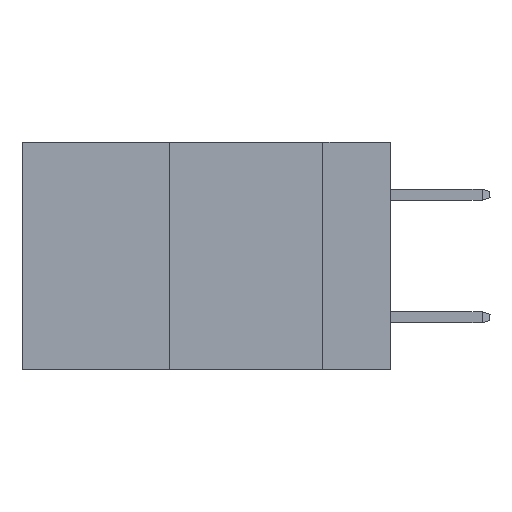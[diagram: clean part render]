
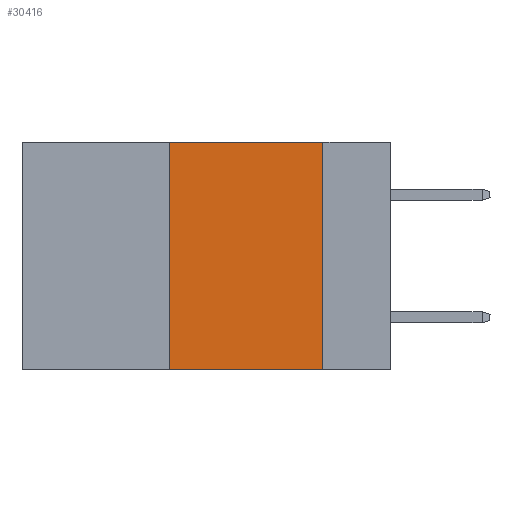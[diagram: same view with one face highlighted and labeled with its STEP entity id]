
A CAD part, left-side view. The second image highlights one B-rep face of the part: STEP entity #30416.
In plain terms, the highlighted planar face has unit normal (-1, 0, 0).
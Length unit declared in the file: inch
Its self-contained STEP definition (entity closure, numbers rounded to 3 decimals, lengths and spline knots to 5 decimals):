
#1868 = CARTESIAN_POINT ( 'NONE',  ( 0., 0.11, 0. ) ) ;
#5087 = DIRECTION ( 'NONE',  ( 1., 0., 0. ) ) ;
#5675 = CARTESIAN_POINT ( 'NONE',  ( 0., 0.6, 0. ) ) ;
#8680 = DIRECTION ( 'NONE',  ( 0., 0., -1. ) ) ;
#9244 = CARTESIAN_POINT ( 'NONE',  ( 0., 0.6, 0. ) ) ;
#10865 = DIRECTION ( 'NONE',  ( 0., -1., 0. ) ) ;
#11675 = ORIENTED_EDGE ( 'NONE', *, *, #19535, .T. ) ;
#11984 = DIRECTION ( 'NONE',  ( 0., 0., -1. ) ) ;
#12924 = ORIENTED_EDGE ( 'NONE', *, *, #38680, .F. ) ;
#15385 = VECTOR ( 'NONE', #33430, 39.37008 ) ;
#16258 = VERTEX_POINT ( 'NONE', #24837 ) ;
#16572 = EDGE_CURVE ( 'NONE', #40234, #34089, #17616, .T. ) ;
#17616 = LINE ( 'NONE', #18997, #23448 ) ;
#18564 = AXIS2_PLACEMENT_3D ( 'NONE', #5675, #5087, #8680 ) ;
#18851 = FACE_OUTER_BOUND ( 'NONE', #28103, .T. ) ;
#18997 = CARTESIAN_POINT ( 'NONE',  ( 0., 0.36, 0. ) ) ;
#19535 = EDGE_CURVE ( 'NONE', #40234, #16258, #28374, .T. ) ;
#21139 = VERTEX_POINT ( 'NONE', #42119 ) ;
#21754 = VECTOR ( 'NONE', #11984, 39.37008 ) ;
#22454 = DIRECTION ( 'NONE',  ( 0., 0., 1. ) ) ;
#23448 = VECTOR ( 'NONE', #22454, 39.37008 ) ;
#23843 = LINE ( 'NONE', #1868, #21754 ) ;
#24837 = CARTESIAN_POINT ( 'NONE',  ( 0., 0.11, -0.37 ) ) ;
#25676 = VECTOR ( 'NONE', #10865, 39.37008 ) ;
#28103 = EDGE_LOOP ( 'NONE', ( #12924, #36488, #29905, #11675 ) ) ;
#28374 = LINE ( 'NONE', #41032, #25676 ) ;
#29016 = PLANE ( 'NONE',  #18564 ) ;
#29905 = ORIENTED_EDGE ( 'NONE', *, *, #16572, .F. ) ;
#30416 = ADVANCED_FACE ( 'NONE', ( #18851 ), #29016, .F. ) ;
#32951 = CARTESIAN_POINT ( 'NONE',  ( 0., 0.36, -0.37 ) ) ;
#33430 = DIRECTION ( 'NONE',  ( 0., -1., 0. ) ) ;
#34089 = VERTEX_POINT ( 'NONE', #39034 ) ;
#35169 = LINE ( 'NONE', #9244, #15385 ) ;
#36488 = ORIENTED_EDGE ( 'NONE', *, *, #41362, .F. ) ;
#38680 = EDGE_CURVE ( 'NONE', #21139, #16258, #23843, .T. ) ;
#39034 = CARTESIAN_POINT ( 'NONE',  ( 0., 0.36, 0. ) ) ;
#40234 = VERTEX_POINT ( 'NONE', #32951 ) ;
#41032 = CARTESIAN_POINT ( 'NONE',  ( 0., 0.6, -0.37 ) ) ;
#41362 = EDGE_CURVE ( 'NONE', #34089, #21139, #35169, .T. ) ;
#42119 = CARTESIAN_POINT ( 'NONE',  ( 0., 0.11, 0. ) ) ;
